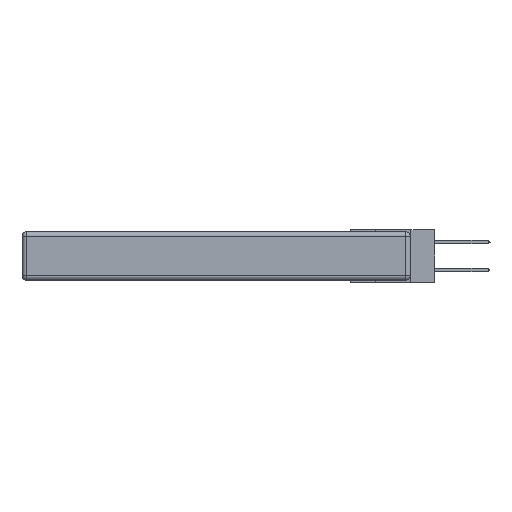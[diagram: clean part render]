
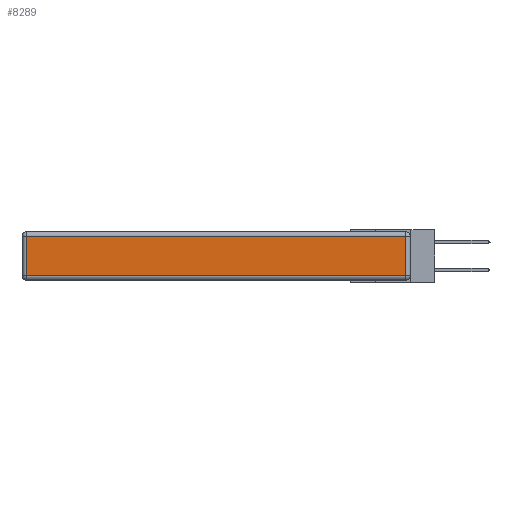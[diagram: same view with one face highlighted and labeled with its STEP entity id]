
A CAD part, left-side view. The second image highlights one B-rep face of the part: STEP entity #8289.
In plain terms, the highlighted planar face has unit normal (-1, 0, 0).
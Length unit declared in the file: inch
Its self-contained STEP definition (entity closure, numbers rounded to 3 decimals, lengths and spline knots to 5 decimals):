
#423 = ORIENTED_EDGE ( 'NONE', *, *, #9221, .T. ) ;
#894 = DIRECTION ( 'NONE',  ( 0., 0., 1. ) ) ;
#1260 = ORIENTED_EDGE ( 'NONE', *, *, #8945, .T. ) ;
#1830 = DIRECTION ( 'NONE',  ( 0., 0., -1. ) ) ;
#3377 = EDGE_CURVE ( 'NONE', #4899, #12607, #9208, .T. ) ;
#4327 = CARTESIAN_POINT ( 'NONE',  ( 0., 0.03, -0.313 ) ) ;
#4792 = CARTESIAN_POINT ( 'NONE',  ( 0., 0., -0.313 ) ) ;
#4899 = VERTEX_POINT ( 'NONE', #7906 ) ;
#5132 = CARTESIAN_POINT ( 'NONE',  ( 0., 0.03, -0.343 ) ) ;
#7702 = EDGE_CURVE ( 'NONE', #12607, #8117, #23520, .T. ) ;
#7906 = CARTESIAN_POINT ( 'NONE',  ( 0., 2.72, -0.03 ) ) ;
#7947 = VERTEX_POINT ( 'NONE', #9798 ) ;
#8117 = VERTEX_POINT ( 'NONE', #4327 ) ;
#8289 = ADVANCED_FACE ( 'NONE', ( #12556 ), #19984, .T. ) ;
#8599 = EDGE_LOOP ( 'NONE', ( #9918, #423, #1260, #9987 ) ) ;
#8945 = EDGE_CURVE ( 'NONE', #7947, #4899, #13425, .T. ) ;
#9208 = LINE ( 'NONE', #23450, #13737 ) ;
#9221 = EDGE_CURVE ( 'NONE', #8117, #7947, #24968, .T. ) ;
#9798 = CARTESIAN_POINT ( 'NONE',  ( 0., 0.03, -0.03 ) ) ;
#9918 = ORIENTED_EDGE ( 'NONE', *, *, #7702, .T. ) ;
#9987 = ORIENTED_EDGE ( 'NONE', *, *, #3377, .T. ) ;
#11027 = DIRECTION ( 'NONE',  ( 0., 0., 1. ) ) ;
#12384 = CARTESIAN_POINT ( 'NONE',  ( 0., 0., -0.343 ) ) ;
#12442 = DIRECTION ( 'NONE',  ( 0., -1., 0. ) ) ;
#12465 = DIRECTION ( 'NONE',  ( -1., 0., 0. ) ) ;
#12556 = FACE_OUTER_BOUND ( 'NONE', #8599, .T. ) ;
#12607 = VERTEX_POINT ( 'NONE', #16324 ) ;
#13129 = VECTOR ( 'NONE', #15298, 39.37008 ) ;
#13425 = LINE ( 'NONE', #23648, #13129 ) ;
#13737 = VECTOR ( 'NONE', #1830, 39.37008 ) ;
#14013 = VECTOR ( 'NONE', #11027, 39.37008 ) ;
#15002 = AXIS2_PLACEMENT_3D ( 'NONE', #12384, #12465, #894 ) ;
#15298 = DIRECTION ( 'NONE',  ( 0., 1., 0. ) ) ;
#15941 = VECTOR ( 'NONE', #12442, 39.37008 ) ;
#16324 = CARTESIAN_POINT ( 'NONE',  ( 0., 2.72, -0.313 ) ) ;
#19984 = PLANE ( 'NONE',  #15002 ) ;
#23450 = CARTESIAN_POINT ( 'NONE',  ( 0., 2.72, -0.343 ) ) ;
#23520 = LINE ( 'NONE', #4792, #15941 ) ;
#23648 = CARTESIAN_POINT ( 'NONE',  ( 0., 2.75, -0.03 ) ) ;
#24968 = LINE ( 'NONE', #5132, #14013 ) ;
